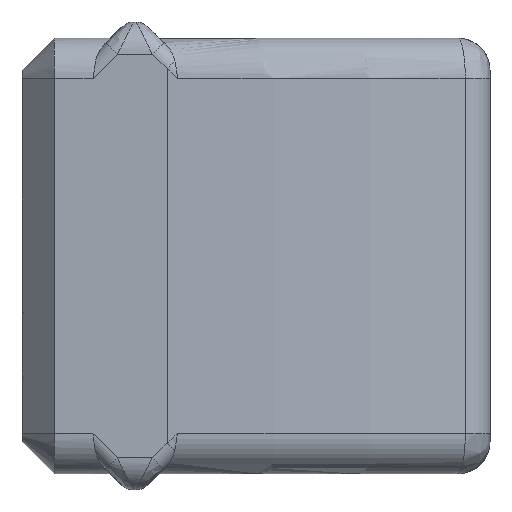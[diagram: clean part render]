
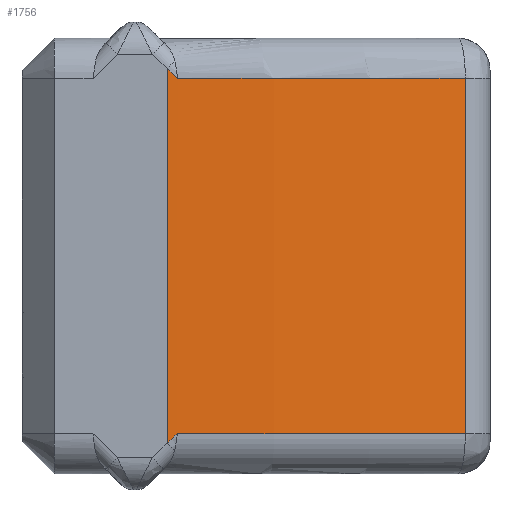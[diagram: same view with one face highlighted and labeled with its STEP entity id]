
A CAD part, left-side view. The second image highlights one B-rep face of the part: STEP entity #1756.
In plain terms, the highlighted cylindrical face has radius 98.27 mm (diameter 196.54 mm), a partial arc.
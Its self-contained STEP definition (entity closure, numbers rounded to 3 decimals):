
#86=CIRCLE('',#1930,98.27);
#87=CIRCLE('',#1931,98.27);
#107=ELLIPSE('',#1920,138.269,98.27);
#110=ELLIPSE('',#1928,138.269,98.27);
#133=CYLINDRICAL_SURFACE('',#1929,98.27);
#262=FACE_OUTER_BOUND('',#367,.T.);
#367=EDGE_LOOP('',(#1555,#1556,#1557,#1558,#1559,#1560,#1561,#1562));
#487=LINE('',#3689,#618);
#503=LINE('',#4082,#634);
#618=VECTOR('',#2230,10.);
#634=VECTOR('',#2352,10.);
#692=B_SPLINE_CURVE_WITH_KNOTS('',3,(#3862,#3863,#3864,#3865,#3866,#3867,
#3868,#3869),.UNSPECIFIED.,.F.,.F.,(4,2,2,4),(1.53,1.531,
1.533,1.534),.UNSPECIFIED.);
#698=B_SPLINE_CURVE_WITH_KNOTS('',3,(#4030,#4031,#4032,#4033,#4034,#4035,
#4036,#4037),.UNSPECIFIED.,.F.,.F.,(4,2,2,4),(1.525,1.526,
1.527,1.528),.UNSPECIFIED.);
#830=VERTEX_POINT('',#3686);
#831=VERTEX_POINT('',#3688);
#852=VERTEX_POINT('',#3861);
#854=VERTEX_POINT('',#3912);
#855=VERTEX_POINT('',#4003);
#857=VERTEX_POINT('',#4054);
#858=VERTEX_POINT('',#4079);
#859=VERTEX_POINT('',#4081);
#1047=EDGE_CURVE('',#830,#831,#487,.T.);
#1090=EDGE_CURVE('',#852,#830,#692,.T.);
#1094=EDGE_CURVE('',#854,#852,#107,.T.);
#1101=EDGE_CURVE('',#831,#855,#698,.T.);
#1102=EDGE_CURVE('',#855,#857,#110,.T.);
#1104=EDGE_CURVE('',#858,#854,#86,.T.);
#1105=EDGE_CURVE('',#859,#858,#503,.T.);
#1106=EDGE_CURVE('',#857,#859,#87,.T.);
#1555=ORIENTED_EDGE('',*,*,#1090,.F.);
#1556=ORIENTED_EDGE('',*,*,#1094,.F.);
#1557=ORIENTED_EDGE('',*,*,#1104,.F.);
#1558=ORIENTED_EDGE('',*,*,#1105,.F.);
#1559=ORIENTED_EDGE('',*,*,#1106,.F.);
#1560=ORIENTED_EDGE('',*,*,#1102,.F.);
#1561=ORIENTED_EDGE('',*,*,#1101,.F.);
#1562=ORIENTED_EDGE('',*,*,#1047,.F.);
#1756=ADVANCED_FACE('',(#262),#133,.T.);
#1920=AXIS2_PLACEMENT_3D('',#3935,#2330,#2331);
#1928=AXIS2_PLACEMENT_3D('',#4055,#2346,#2347);
#1929=AXIS2_PLACEMENT_3D('',#4078,#2348,#2349);
#1930=AXIS2_PLACEMENT_3D('',#4080,#2350,#2351);
#1931=AXIS2_PLACEMENT_3D('',#4083,#2353,#2354);
#2230=DIRECTION('',(0.,0.,1.));
#2330=DIRECTION('center_axis',(0.,-0.703,
-0.711));
#2331=DIRECTION('ref_axis',(0.,-0.711,0.703));
#2346=DIRECTION('center_axis',(0.,-0.703,
0.711));
#2347=DIRECTION('ref_axis',(0.,-0.711,-0.703));
#2348=DIRECTION('center_axis',(0.,0.,1.));
#2349=DIRECTION('ref_axis',(-0.999,0.046,0.));
#2350=DIRECTION('center_axis',(0.,0.,-1.));
#2351=DIRECTION('ref_axis',(-0.989,-0.148,0.));
#2352=DIRECTION('',(0.,0.,-1.));
#2353=DIRECTION('center_axis',(0.,0.,1.));
#2354=DIRECTION('ref_axis',(-0.989,-0.148,0.));
#3686=CARTESIAN_POINT('',(-19.,-27.,-0.071));
#3688=CARTESIAN_POINT('',(-19.,-27.,23.086));
#3689=CARTESIAN_POINT('',(-19.,-27.,0.));
#3861=CARTESIAN_POINT('',(-18.999,-27.011,-0.105));
#3862=CARTESIAN_POINT('Ctrl Pts',(-18.999,-27.011,-0.105));
#3863=CARTESIAN_POINT('Ctrl Pts',(-19.,-27.01,-0.104));
#3864=CARTESIAN_POINT('Ctrl Pts',(-19.,-27.009,-0.102));
#3865=CARTESIAN_POINT('Ctrl Pts',(-19.,-27.005,-0.096));
#3866=CARTESIAN_POINT('Ctrl Pts',(-19.,-27.003,-0.091));
#3867=CARTESIAN_POINT('Ctrl Pts',(-19.,-27.,-0.081));
#3868=CARTESIAN_POINT('Ctrl Pts',(-19.,-27.,-0.076));
#3869=CARTESIAN_POINT('Ctrl Pts',(-19.,-27.,-0.071));
#3912=CARTESIAN_POINT('',(-18.969,-27.623,0.5));
#3935=CARTESIAN_POINT('Origin',(79.167,-22.5,-4.571));
#4003=CARTESIAN_POINT('',(-18.999,-27.011,23.12));
#4030=CARTESIAN_POINT('Ctrl Pts',(-19.,-27.,23.086));
#4031=CARTESIAN_POINT('Ctrl Pts',(-19.,-27.,23.091));
#4032=CARTESIAN_POINT('Ctrl Pts',(-19.,-27.,23.096));
#4033=CARTESIAN_POINT('Ctrl Pts',(-19.,-27.003,23.106));
#4034=CARTESIAN_POINT('Ctrl Pts',(-19.,-27.005,23.111));
#4035=CARTESIAN_POINT('Ctrl Pts',(-19.,-27.009,23.117));
#4036=CARTESIAN_POINT('Ctrl Pts',(-19.,-27.01,23.119));
#4037=CARTESIAN_POINT('Ctrl Pts',(-18.999,-27.011,23.12));
#4054=CARTESIAN_POINT('',(-18.969,-27.638,22.5));
#4055=CARTESIAN_POINT('Origin',(79.167,-22.5,27.586));
#4078=CARTESIAN_POINT('Origin',(79.167,-22.5,0.));
#4079=CARTESIAN_POINT('',(-16.381,-45.467,0.5));
#4080=CARTESIAN_POINT('Origin',(79.167,-22.5,0.5));
#4081=CARTESIAN_POINT('',(-16.381,-45.467,22.5));
#4082=CARTESIAN_POINT('',(-16.381,-45.467,0.));
#4083=CARTESIAN_POINT('Origin',(79.167,-22.5,22.5));
